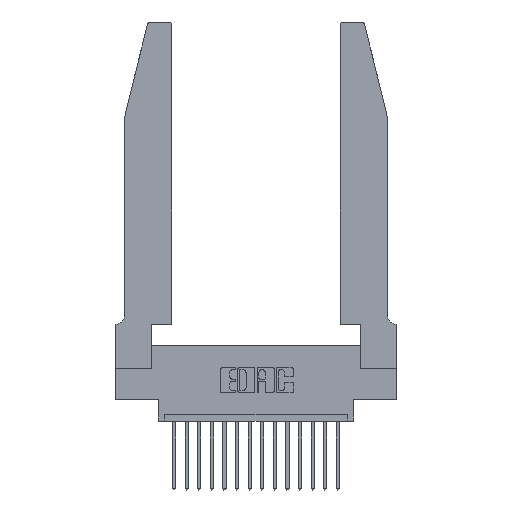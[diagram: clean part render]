
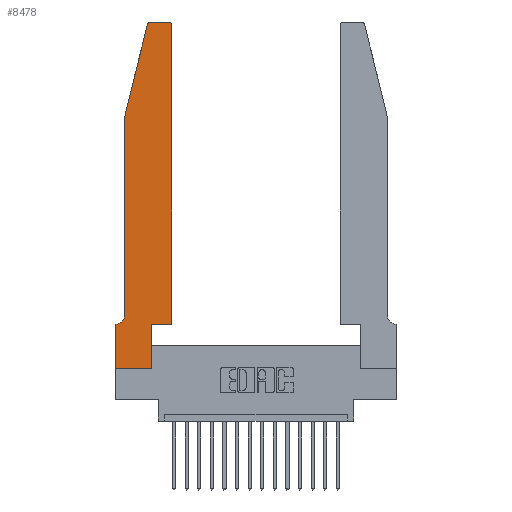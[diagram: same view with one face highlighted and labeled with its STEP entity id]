
A CAD part, top view. The second image highlights one B-rep face of the part: STEP entity #8478.
In plain terms, the highlighted planar face has unit normal (0, 0, 1).
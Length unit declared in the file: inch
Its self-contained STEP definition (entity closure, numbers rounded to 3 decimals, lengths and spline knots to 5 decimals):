
#14 = CARTESIAN_POINT ( 'NONE',  ( 0.4505, 2.72, 0.37 ) ) ;
#74 = VERTEX_POINT ( 'NONE', #16639 ) ;
#118 = CIRCLE ( 'NONE', #14617, 0.03 ) ;
#148 = ORIENTED_EDGE ( 'NONE', *, *, #17709, .T. ) ;
#431 = CARTESIAN_POINT ( 'NONE',  ( 0.0755, 0.42, 0.37 ) ) ;
#712 = ORIENTED_EDGE ( 'NONE', *, *, #13885, .T. ) ;
#834 = VERTEX_POINT ( 'NONE', #12130 ) ;
#1732 = AXIS2_PLACEMENT_3D ( 'NONE', #4883, #12331, #3327 ) ;
#1736 = LINE ( 'NONE', #15951, #3373 ) ;
#1895 = FACE_OUTER_BOUND ( 'NONE', #3766, .T. ) ;
#2034 = CARTESIAN_POINT ( 'NONE',  ( 0.2605, 2.75, 0.37 ) ) ;
#2076 = EDGE_CURVE ( 'NONE', #12933, #5694, #1736, .T. ) ;
#2372 = LINE ( 'NONE', #10391, #3521 ) ;
#2459 = DIRECTION ( 'NONE',  ( 0., 1., 0. ) ) ;
#2636 = CARTESIAN_POINT ( 'NONE',  ( 0.284, 2.72, 0.37 ) ) ;
#3026 = ORIENTED_EDGE ( 'NONE', *, *, #17843, .T. ) ;
#3327 = DIRECTION ( 'NONE',  ( -1., 0., 0. ) ) ;
#3373 = VECTOR ( 'NONE', #14257, 39.37008 ) ;
#3435 = LINE ( 'NONE', #12155, #13415 ) ;
#3521 = VECTOR ( 'NONE', #16446, 39.37008 ) ;
#3766 = EDGE_LOOP ( 'NONE', ( #148, #14854, #12845, #3026, #5353, #12956, #9556, #18117, #712, #18254, #19197, #5676 ) ) ;
#4382 = CARTESIAN_POINT ( 'NONE',  ( 0.4505, 0.35, 0.37 ) ) ;
#4707 = VERTEX_POINT ( 'NONE', #11969 ) ;
#4745 = EDGE_CURVE ( 'NONE', #16882, #12299, #8842, .T. ) ;
#4883 = CARTESIAN_POINT ( 'NONE',  ( 0.0055, 0.42, 0.37 ) ) ;
#4932 = CARTESIAN_POINT ( 'NONE',  ( 0.4205, 2.75, 0.37 ) ) ;
#5060 = CIRCLE ( 'NONE', #5216, 0.03 ) ;
#5187 = VERTEX_POINT ( 'NONE', #14 ) ;
#5216 = AXIS2_PLACEMENT_3D ( 'NONE', #16764, #11759, #9494 ) ;
#5353 = ORIENTED_EDGE ( 'NONE', *, *, #14522, .T. ) ;
#5557 = VERTEX_POINT ( 'NONE', #4932 ) ;
#5676 = ORIENTED_EDGE ( 'NONE', *, *, #13992, .T. ) ;
#5690 = VECTOR ( 'NONE', #18879, 39.37008 ) ;
#5694 = VERTEX_POINT ( 'NONE', #11077 ) ;
#5819 = VECTOR ( 'NONE', #18013, 39.37008 ) ;
#5864 = LINE ( 'NONE', #18834, #11414 ) ;
#6392 = EDGE_CURVE ( 'NONE', #4707, #834, #118, .T. ) ;
#6526 = CARTESIAN_POINT ( 'NONE',  ( 0.0755, 2., 0.37 ) ) ;
#6926 = EDGE_CURVE ( 'NONE', #74, #7908, #8954, .T. ) ;
#7908 = VERTEX_POINT ( 'NONE', #4382 ) ;
#7957 = AXIS2_PLACEMENT_3D ( 'NONE', #9554, #17575, #14441 ) ;
#8478 = ADVANCED_FACE ( 'NONE', ( #1895 ), #18449, .T. ) ;
#8639 = EDGE_CURVE ( 'NONE', #12299, #12933, #2372, .T. ) ;
#8842 = LINE ( 'NONE', #9203, #5819 ) ;
#8954 = LINE ( 'NONE', #14480, #5690 ) ;
#9203 = CARTESIAN_POINT ( 'NONE',  ( 0.0755, 0.35, 0.37 ) ) ;
#9494 = DIRECTION ( 'NONE',  ( 1., 0., 0. ) ) ;
#9554 = CARTESIAN_POINT ( 'NONE',  ( 0., 0.35, 0.37 ) ) ;
#9556 = ORIENTED_EDGE ( 'NONE', *, *, #8639, .T. ) ;
#10168 = CARTESIAN_POINT ( 'NONE',  ( 0., 0.35, 0.37 ) ) ;
#10391 = CARTESIAN_POINT ( 'NONE',  ( 0., 0., 0.37 ) ) ;
#10490 = EDGE_CURVE ( 'NONE', #834, #17064, #15503, .T. ) ;
#10938 = DIRECTION ( 'NONE',  ( -0.239, -0.971, 0. ) ) ;
#11077 = CARTESIAN_POINT ( 'NONE',  ( 0.2865, 0., 0.37 ) ) ;
#11414 = VECTOR ( 'NONE', #11619, 39.37008 ) ;
#11619 = DIRECTION ( 'NONE',  ( 0., -1., 0. ) ) ;
#11759 = DIRECTION ( 'NONE',  ( 0., 0., 1. ) ) ;
#11873 = VECTOR ( 'NONE', #14098, 39.37008 ) ;
#11969 = CARTESIAN_POINT ( 'NONE',  ( 0.284, 2.75, 0.37 ) ) ;
#12130 = CARTESIAN_POINT ( 'NONE',  ( 0.25487, 2.72718, 0.37 ) ) ;
#12155 = CARTESIAN_POINT ( 'NONE',  ( 0.2865, 0.35, 0.37 ) ) ;
#12248 = LINE ( 'NONE', #13714, #17377 ) ;
#12299 = VERTEX_POINT ( 'NONE', #10168 ) ;
#12331 = DIRECTION ( 'NONE',  ( 0., 0., -1. ) ) ;
#12845 = ORIENTED_EDGE ( 'NONE', *, *, #10490, .T. ) ;
#12933 = VERTEX_POINT ( 'NONE', #16723 ) ;
#12956 = ORIENTED_EDGE ( 'NONE', *, *, #4745, .T. ) ;
#12958 = DIRECTION ( 'NONE',  ( 0., 0., 1. ) ) ;
#13415 = VECTOR ( 'NONE', #15196, 39.37008 ) ;
#13714 = CARTESIAN_POINT ( 'NONE',  ( 0.4505, 0.35, 0.37 ) ) ;
#13885 = EDGE_CURVE ( 'NONE', #5694, #74, #3435, .T. ) ;
#13889 = EDGE_CURVE ( 'NONE', #7908, #5187, #12248, .T. ) ;
#13992 = EDGE_CURVE ( 'NONE', #5187, #5557, #5060, .T. ) ;
#14098 = DIRECTION ( 'NONE',  ( -1., 0., 0. ) ) ;
#14109 = VECTOR ( 'NONE', #10938, 39.37008 ) ;
#14257 = DIRECTION ( 'NONE',  ( 1., 0., 0. ) ) ;
#14441 = DIRECTION ( 'NONE',  ( 1., 0., 0. ) ) ;
#14480 = CARTESIAN_POINT ( 'NONE',  ( 0.4505, 0.35, 0.37 ) ) ;
#14497 = DIRECTION ( 'NONE',  ( 1., 0., 0. ) ) ;
#14522 = EDGE_CURVE ( 'NONE', #15765, #16882, #14577, .T. ) ;
#14577 = CIRCLE ( 'NONE', #1732, 0.07 ) ;
#14617 = AXIS2_PLACEMENT_3D ( 'NONE', #2636, #12958, #14497 ) ;
#14689 = LINE ( 'NONE', #2034, #11873 ) ;
#14854 = ORIENTED_EDGE ( 'NONE', *, *, #6392, .T. ) ;
#15196 = DIRECTION ( 'NONE',  ( 0., 1., 0. ) ) ;
#15503 = LINE ( 'NONE', #6526, #14109 ) ;
#15758 = CARTESIAN_POINT ( 'NONE',  ( 0.0055, 0.35, 0.37 ) ) ;
#15765 = VERTEX_POINT ( 'NONE', #431 ) ;
#15951 = CARTESIAN_POINT ( 'NONE',  ( 0., 0., 0.37 ) ) ;
#16446 = DIRECTION ( 'NONE',  ( 0., -1., 0. ) ) ;
#16639 = CARTESIAN_POINT ( 'NONE',  ( 0.2865, 0.35, 0.37 ) ) ;
#16723 = CARTESIAN_POINT ( 'NONE',  ( 0., 0., 0.37 ) ) ;
#16764 = CARTESIAN_POINT ( 'NONE',  ( 0.4205, 2.72, 0.37 ) ) ;
#16882 = VERTEX_POINT ( 'NONE', #15758 ) ;
#17064 = VERTEX_POINT ( 'NONE', #17717 ) ;
#17377 = VECTOR ( 'NONE', #2459, 39.37008 ) ;
#17575 = DIRECTION ( 'NONE',  ( 0., 0., 1. ) ) ;
#17709 = EDGE_CURVE ( 'NONE', #5557, #4707, #14689, .T. ) ;
#17717 = CARTESIAN_POINT ( 'NONE',  ( 0.0755, 2., 0.37 ) ) ;
#17843 = EDGE_CURVE ( 'NONE', #17064, #15765, #5864, .T. ) ;
#18013 = DIRECTION ( 'NONE',  ( -1., 0., 0. ) ) ;
#18117 = ORIENTED_EDGE ( 'NONE', *, *, #2076, .T. ) ;
#18254 = ORIENTED_EDGE ( 'NONE', *, *, #6926, .T. ) ;
#18449 = PLANE ( 'NONE',  #7957 ) ;
#18834 = CARTESIAN_POINT ( 'NONE',  ( 0.0755, 2., 0.37 ) ) ;
#18879 = DIRECTION ( 'NONE',  ( 1., 0., 0. ) ) ;
#19197 = ORIENTED_EDGE ( 'NONE', *, *, #13889, .T. ) ;
